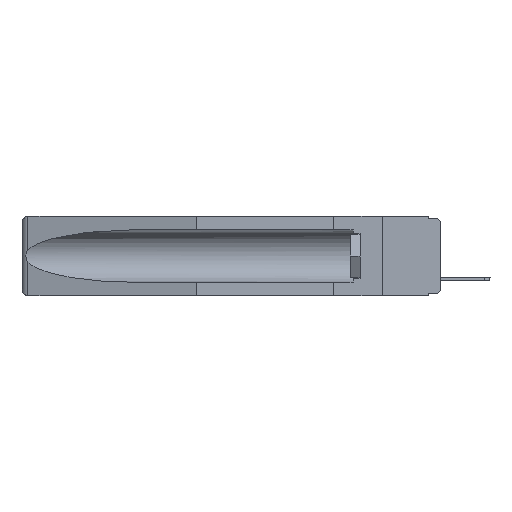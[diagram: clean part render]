
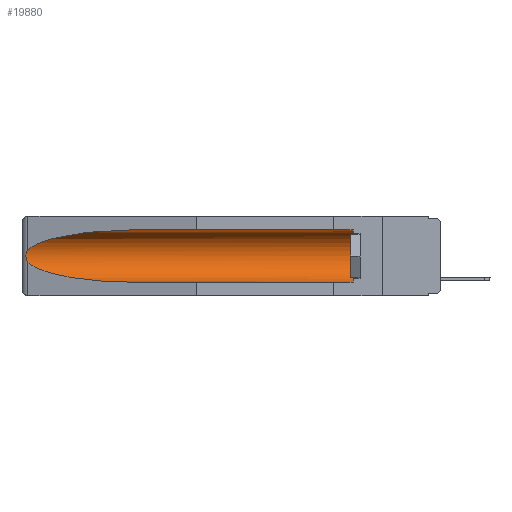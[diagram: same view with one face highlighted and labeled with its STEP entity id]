
A CAD part, left-side view. The second image highlights one B-rep face of the part: STEP entity #19880.
In plain terms, the highlighted cylindrical face has radius 2.857 mm (diameter 5.715 mm), a partial arc.
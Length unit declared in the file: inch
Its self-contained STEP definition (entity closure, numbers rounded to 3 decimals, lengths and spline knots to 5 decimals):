
#707 = VECTOR ( 'NONE', #16458, 39.37008 ) ;
#1571 = ORIENTED_EDGE ( 'NONE', *, *, #17196, .T. ) ;
#1813 = CARTESIAN_POINT ( 'NONE',  ( 0.26597, 1.52961, -0.15275 ) ) ;
#1937 = CARTESIAN_POINT ( 'NONE',  ( 0.26655, 1.53094, -0.18657 ) ) ;
#2600 =( BOUNDED_CURVE ( )  B_SPLINE_CURVE ( 3, ( #9960, #10210, #19424, #4813 ),
 .UNSPECIFIED., .F., .F. ) 
 B_SPLINE_CURVE_WITH_KNOTS ( ( 4, 4 ),
 ( 0.1948, 1.5708 ),
 .UNSPECIFIED. ) 
 CURVE ( )  GEOMETRIC_REPRESENTATION_ITEM ( )  RATIONAL_B_SPLINE_CURVE ( ( 1., 0.848, 0.848, 1. ) ) 
 REPRESENTATION_ITEM ( '' )  );
#2903 = ORIENTED_EDGE ( 'NONE', *, *, #21784, .T. ) ;
#3113 = CARTESIAN_POINT ( 'NONE',  ( 0.155, 1.07973, -0.284 ) ) ;
#3218 = DIRECTION ( 'NONE',  ( 0., 1., 0. ) ) ;
#3581 = CARTESIAN_POINT ( 'NONE',  ( 0.155, 0.126, -0.059 ) ) ;
#4672 = CARTESIAN_POINT ( 'NONE',  ( 0.26537, 1.52718, -0.14972 ) ) ;
#4813 = CARTESIAN_POINT ( 'NONE',  ( 0.155, 1.07973, -0.284 ) ) ;
#5284 = CARTESIAN_POINT ( 'NONE',  ( 0.2673, 1.53269, -0.17917 ) ) ;
#5811 = CARTESIAN_POINT ( 'NONE',  ( 0.26537, 1.52718, -0.14972 ) ) ;
#6233 = ORIENTED_EDGE ( 'NONE', *, *, #10432, .T. ) ;
#6308 = CARTESIAN_POINT ( 'NONE',  ( 0.155, 0.126, -0.284 ) ) ;
#7132 = CARTESIAN_POINT ( 'NONE',  ( 0.26597, 1.5296, -0.19026 ) ) ;
#7140 = AXIS2_PLACEMENT_3D ( 'NONE', #20307, #22058, #12755 ) ;
#7146 = VERTEX_POINT ( 'NONE', #6308 ) ;
#7370 = CARTESIAN_POINT ( 'NONE',  ( 0.26537, 1.52718, -0.14972 ) ) ;
#8139 = CARTESIAN_POINT ( 'NONE',  ( 0.155, 1.07973, -0.059 ) ) ;
#8473 = EDGE_CURVE ( 'NONE', #12090, #8978, #22075, .T. ) ;
#8789 = FACE_OUTER_BOUND ( 'NONE', #11405, .T. ) ;
#8898 = DIRECTION ( 'NONE',  ( 0., 0., 1. ) ) ;
#8978 = VERTEX_POINT ( 'NONE', #4672 ) ;
#9326 = CARTESIAN_POINT ( 'NONE',  ( 0.26537, 1.52718, -0.19328 ) ) ;
#9442 = CARTESIAN_POINT ( 'NONE',  ( 0.2673, 1.5327, -0.16383 ) ) ;
#9960 = CARTESIAN_POINT ( 'NONE',  ( 0.26537, 1.52718, -0.19328 ) ) ;
#10007 = ORIENTED_EDGE ( 'NONE', *, *, #8473, .T. ) ;
#10031 = VERTEX_POINT ( 'NONE', #3581 ) ;
#10210 = CARTESIAN_POINT ( 'NONE',  ( 0.25451, 1.48313, -0.24835 ) ) ;
#10432 = EDGE_CURVE ( 'NONE', #8978, #18467, #12057, .T. ) ;
#11024 = ORIENTED_EDGE ( 'NONE', *, *, #21402, .T. ) ;
#11405 = EDGE_LOOP ( 'NONE', ( #10007, #6233, #2903, #13610, #1571, #11024 ) ) ;
#11483 = CARTESIAN_POINT ( 'NONE',  ( 0.26537, 1.52718, -0.19328 ) ) ;
#12057 = B_SPLINE_CURVE_WITH_KNOTS ( 'NONE', 3,
 ( #7370, #1813, #16549, #9442, #24254, #14572, #5284, #1937, #7132, #9326 ),
 .UNSPECIFIED., .F., .F.,
 ( 4, 2, 2, 2, 4 ),
 ( 0., 0.00029, 0.00058, 0.00087, 0.00117 ),
 .UNSPECIFIED. ) ;
#12090 = VERTEX_POINT ( 'NONE', #15373 ) ;
#12755 = DIRECTION ( 'NONE',  ( 0., 0., 1. ) ) ;
#12775 = DIRECTION ( 'NONE',  ( 0., 1., 0. ) ) ;
#13610 = ORIENTED_EDGE ( 'NONE', *, *, #21482, .F. ) ;
#14572 = CARTESIAN_POINT ( 'NONE',  ( 0.2675, 1.53308, -0.17534 ) ) ;
#14635 = CYLINDRICAL_SURFACE ( 'NONE', #20248, 0.1125 ) ;
#14765 = CARTESIAN_POINT ( 'NONE',  ( 0.155, -0.30754, -0.1715 ) ) ;
#14937 = VERTEX_POINT ( 'NONE', #3113 ) ;
#15373 = CARTESIAN_POINT ( 'NONE',  ( 0.155, 1.07973, -0.059 ) ) ;
#16126 = VECTOR ( 'NONE', #3218, 39.37008 ) ;
#16458 = DIRECTION ( 'NONE',  ( 0., 1., 0. ) ) ;
#16549 = CARTESIAN_POINT ( 'NONE',  ( 0.26654, 1.53092, -0.15636 ) ) ;
#17196 = EDGE_CURVE ( 'NONE', #7146, #10031, #23384, .T. ) ;
#18211 = LINE ( 'NONE', #20427, #707 ) ;
#18467 = VERTEX_POINT ( 'NONE', #11483 ) ;
#18710 = LINE ( 'NONE', #22424, #16126 ) ;
#19312 = CARTESIAN_POINT ( 'NONE',  ( 0.21114, 1.30732, -0.059 ) ) ;
#19424 = CARTESIAN_POINT ( 'NONE',  ( 0.21114, 1.30732, -0.284 ) ) ;
#19880 = ADVANCED_FACE ( 'NONE', ( #8789 ), #14635, .F. ) ;
#20248 = AXIS2_PLACEMENT_3D ( 'NONE', #14765, #12775, #8898 ) ;
#20307 = CARTESIAN_POINT ( 'NONE',  ( 0.155, 0.126, -0.1715 ) ) ;
#20427 = CARTESIAN_POINT ( 'NONE',  ( 0.155, -0.30754, -0.059 ) ) ;
#21185 = CARTESIAN_POINT ( 'NONE',  ( 0.25451, 1.48313, -0.09465 ) ) ;
#21402 = EDGE_CURVE ( 'NONE', #10031, #12090, #18211, .T. ) ;
#21482 = EDGE_CURVE ( 'NONE', #7146, #14937, #18710, .T. ) ;
#21784 = EDGE_CURVE ( 'NONE', #18467, #14937, #2600, .T. ) ;
#22058 = DIRECTION ( 'NONE',  ( 0., -1., 0. ) ) ;
#22075 =( BOUNDED_CURVE ( )  B_SPLINE_CURVE ( 3, ( #8139, #19312, #21185, #5811 ),
 .UNSPECIFIED., .F., .F. ) 
 B_SPLINE_CURVE_WITH_KNOTS ( ( 4, 4 ),
 ( 4.71239, 6.08839 ),
 .UNSPECIFIED. ) 
 CURVE ( )  GEOMETRIC_REPRESENTATION_ITEM ( )  RATIONAL_B_SPLINE_CURVE ( ( 1., 0.848, 0.848, 1. ) ) 
 REPRESENTATION_ITEM ( '' )  );
#22424 = CARTESIAN_POINT ( 'NONE',  ( 0.155, -0.30754, -0.284 ) ) ;
#23384 = CIRCLE ( 'NONE', #7140, 0.1125 ) ;
#24254 = CARTESIAN_POINT ( 'NONE',  ( 0.2675, 1.53308, -0.16763 ) ) ;
